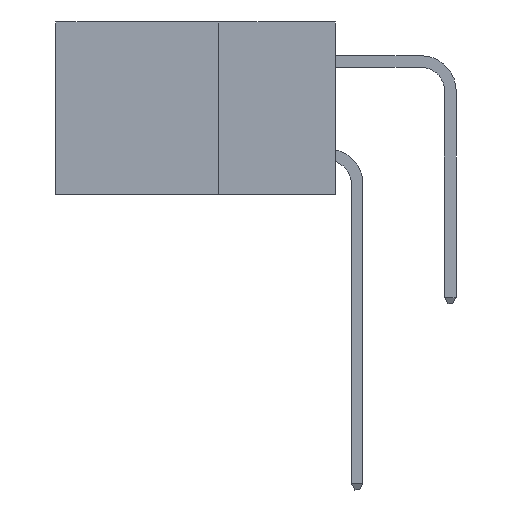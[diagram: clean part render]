
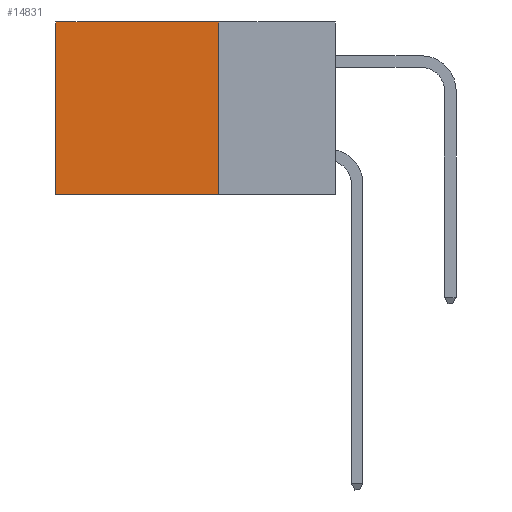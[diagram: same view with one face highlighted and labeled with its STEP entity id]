
A CAD part, left-side view. The second image highlights one B-rep face of the part: STEP entity #14831.
In plain terms, the highlighted planar face has unit normal (-1, 0, 0).
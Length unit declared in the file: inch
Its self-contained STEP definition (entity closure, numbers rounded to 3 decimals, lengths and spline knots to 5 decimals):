
#681 = DIRECTION ( 'NONE',  ( 0., 0., -1. ) ) ;
#902 = CARTESIAN_POINT ( 'NONE',  ( 0.2875, 0.6, -0.37 ) ) ;
#1003 = CARTESIAN_POINT ( 'NONE',  ( 0.2875, 0.25, 0. ) ) ;
#1226 = EDGE_CURVE ( 'NONE', #15543, #10920, #18310, .T. ) ;
#2196 = ORIENTED_EDGE ( 'NONE', *, *, #12825, .T. ) ;
#3190 = DIRECTION ( 'NONE',  ( 1., 0., 0. ) ) ;
#3593 = VECTOR ( 'NONE', #10960, 39.37008 ) ;
#4384 = EDGE_CURVE ( 'NONE', #10920, #11992, #17749, .T. ) ;
#4732 = VECTOR ( 'NONE', #5536, 39.37008 ) ;
#5536 = DIRECTION ( 'NONE',  ( 0., 0., -1. ) ) ;
#5566 = CARTESIAN_POINT ( 'NONE',  ( 0.2875, 0.25, 0. ) ) ;
#5956 = CARTESIAN_POINT ( 'NONE',  ( 0.2875, 0.25, -0.37 ) ) ;
#6780 = AXIS2_PLACEMENT_3D ( 'NONE', #16134, #3190, #16020 ) ;
#6846 = ORIENTED_EDGE ( 'NONE', *, *, #4384, .F. ) ;
#7055 = VECTOR ( 'NONE', #681, 39.37008 ) ;
#7390 = VERTEX_POINT ( 'NONE', #16407 ) ;
#7962 = EDGE_CURVE ( 'NONE', #7390, #11992, #12295, .T. ) ;
#8449 = ORIENTED_EDGE ( 'NONE', *, *, #1226, .F. ) ;
#9990 = ORIENTED_EDGE ( 'NONE', *, *, #7962, .T. ) ;
#10642 = CARTESIAN_POINT ( 'NONE',  ( 0.2875, 0.25, 0. ) ) ;
#10920 = VERTEX_POINT ( 'NONE', #11009 ) ;
#10960 = DIRECTION ( 'NONE',  ( 0., 1., 0. ) ) ;
#11009 = CARTESIAN_POINT ( 'NONE',  ( 0.2875, 0.25, -0.37 ) ) ;
#11602 = EDGE_LOOP ( 'NONE', ( #9990, #6846, #8449, #2196 ) ) ;
#11619 = LINE ( 'NONE', #1003, #3593 ) ;
#11762 = FACE_OUTER_BOUND ( 'NONE', #11602, .T. ) ;
#11992 = VERTEX_POINT ( 'NONE', #902 ) ;
#12295 = LINE ( 'NONE', #17706, #4732 ) ;
#12825 = EDGE_CURVE ( 'NONE', #15543, #7390, #11619, .T. ) ;
#13165 = PLANE ( 'NONE',  #6780 ) ;
#14831 = ADVANCED_FACE ( 'NONE', ( #11762 ), #13165, .F. ) ;
#15543 = VERTEX_POINT ( 'NONE', #5566 ) ;
#16020 = DIRECTION ( 'NONE',  ( 0., 0., -1. ) ) ;
#16134 = CARTESIAN_POINT ( 'NONE',  ( 0.2875, 0.25, 0. ) ) ;
#16407 = CARTESIAN_POINT ( 'NONE',  ( 0.2875, 0.6, 0. ) ) ;
#16879 = VECTOR ( 'NONE', #17354, 39.37008 ) ;
#17354 = DIRECTION ( 'NONE',  ( 0., 1., 0. ) ) ;
#17706 = CARTESIAN_POINT ( 'NONE',  ( 0.2875, 0.6, 0. ) ) ;
#17749 = LINE ( 'NONE', #5956, #16879 ) ;
#18310 = LINE ( 'NONE', #10642, #7055 ) ;
